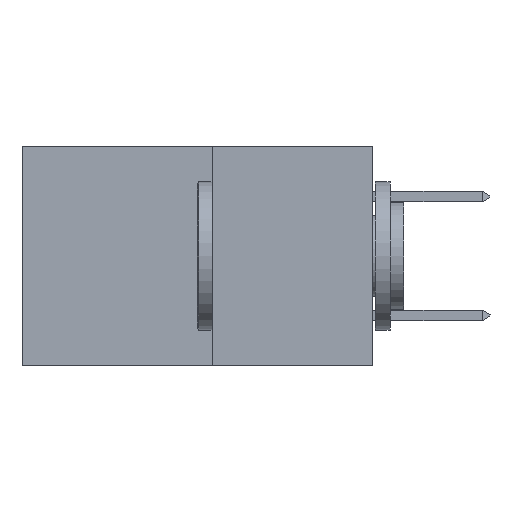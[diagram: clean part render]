
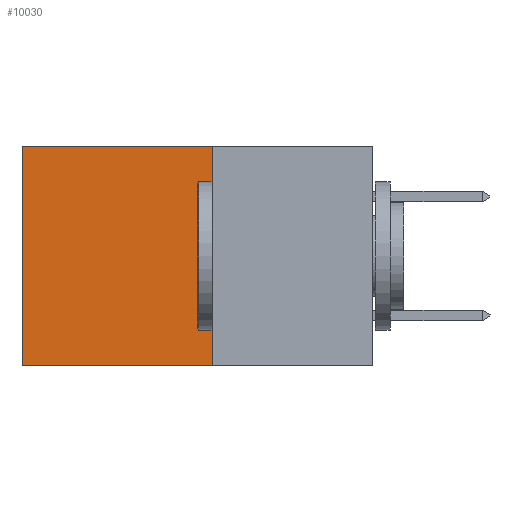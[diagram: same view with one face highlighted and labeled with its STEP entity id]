
A CAD part, left-side view. The second image highlights one B-rep face of the part: STEP entity #10030.
In plain terms, the highlighted planar face has unit normal (-1, 0, 0).
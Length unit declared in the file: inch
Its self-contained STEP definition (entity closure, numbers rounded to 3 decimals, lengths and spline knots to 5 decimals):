
#316 = AXIS2_PLACEMENT_3D ( 'NONE', #16189, #582, #12792 ) ;
#582 = DIRECTION ( 'NONE',  ( 1., 0., 0. ) ) ;
#2116 = ORIENTED_EDGE ( 'NONE', *, *, #5107, .T. ) ;
#2555 = VERTEX_POINT ( 'NONE', #8271 ) ;
#3231 = VECTOR ( 'NONE', #15615, 39.37008 ) ;
#3261 = EDGE_LOOP ( 'NONE', ( #2116, #20630, #3356, #12318 ) ) ;
#3356 = ORIENTED_EDGE ( 'NONE', *, *, #8648, .F. ) ;
#3464 = FACE_OUTER_BOUND ( 'NONE', #3261, .T. ) ;
#4096 = CARTESIAN_POINT ( 'NONE',  ( 0.277, 0.59, -0.37 ) ) ;
#4308 = LINE ( 'NONE', #6841, #3231 ) ;
#5107 = EDGE_CURVE ( 'NONE', #5120, #14126, #18248, .T. ) ;
#5120 = VERTEX_POINT ( 'NONE', #18065 ) ;
#5134 = LINE ( 'NONE', #13969, #9231 ) ;
#5274 = DIRECTION ( 'NONE',  ( 0., 1., 0. ) ) ;
#5435 = VECTOR ( 'NONE', #16294, 39.37008 ) ;
#5462 = CARTESIAN_POINT ( 'NONE',  ( 0.277, 0.27, 0. ) ) ;
#6647 = VECTOR ( 'NONE', #7207, 39.37008 ) ;
#6841 = CARTESIAN_POINT ( 'NONE',  ( 0.277, 0.27, -0.37 ) ) ;
#7207 = DIRECTION ( 'NONE',  ( 0., 1., 0. ) ) ;
#7961 = CARTESIAN_POINT ( 'NONE',  ( 0.277, 0.27, -0.37 ) ) ;
#8271 = CARTESIAN_POINT ( 'NONE',  ( 0.277, 0.27, 0. ) ) ;
#8648 = EDGE_CURVE ( 'NONE', #2555, #19882, #4308, .T. ) ;
#9231 = VECTOR ( 'NONE', #5274, 39.37008 ) ;
#10030 = ADVANCED_FACE ( 'NONE', ( #3464 ), #11035, .F. ) ;
#11035 = PLANE ( 'NONE',  #316 ) ;
#12318 = ORIENTED_EDGE ( 'NONE', *, *, #15048, .T. ) ;
#12792 = DIRECTION ( 'NONE',  ( 0., 0., -1. ) ) ;
#13969 = CARTESIAN_POINT ( 'NONE',  ( 0.277, 0.27, -0.37 ) ) ;
#14126 = VERTEX_POINT ( 'NONE', #18830 ) ;
#15048 = EDGE_CURVE ( 'NONE', #2555, #5120, #20551, .T. ) ;
#15615 = DIRECTION ( 'NONE',  ( 0., 0., -1. ) ) ;
#16189 = CARTESIAN_POINT ( 'NONE',  ( 0.277, 0.27, -0.37 ) ) ;
#16294 = DIRECTION ( 'NONE',  ( 0., 0., -1. ) ) ;
#18065 = CARTESIAN_POINT ( 'NONE',  ( 0.277, 0.59, 0. ) ) ;
#18248 = LINE ( 'NONE', #4096, #5435 ) ;
#18534 = EDGE_CURVE ( 'NONE', #19882, #14126, #5134, .T. ) ;
#18830 = CARTESIAN_POINT ( 'NONE',  ( 0.277, 0.59, -0.37 ) ) ;
#19882 = VERTEX_POINT ( 'NONE', #7961 ) ;
#20551 = LINE ( 'NONE', #5462, #6647 ) ;
#20630 = ORIENTED_EDGE ( 'NONE', *, *, #18534, .F. ) ;
